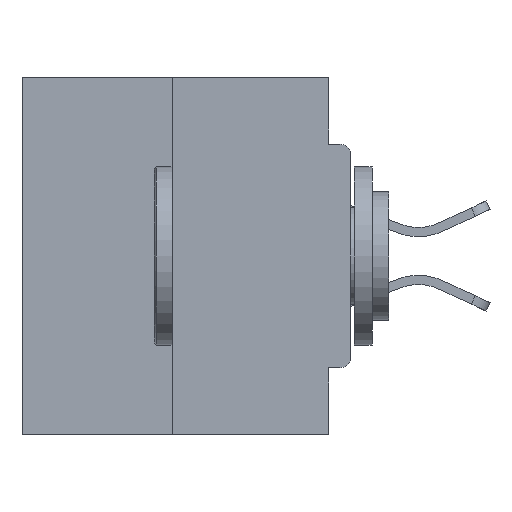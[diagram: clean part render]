
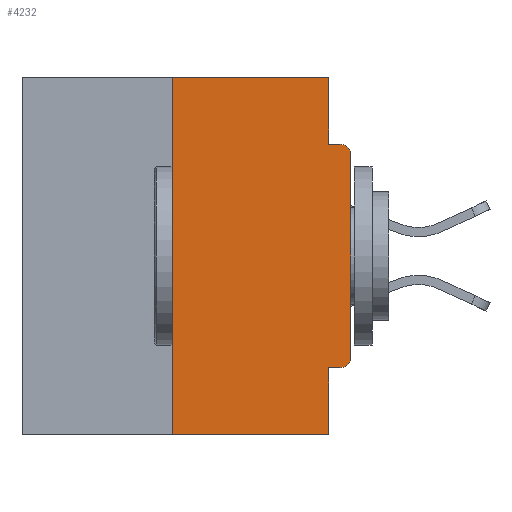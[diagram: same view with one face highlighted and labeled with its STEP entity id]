
A CAD part, left-side view. The second image highlights one B-rep face of the part: STEP entity #4232.
In plain terms, the highlighted planar face has unit normal (-1, 0, 0).
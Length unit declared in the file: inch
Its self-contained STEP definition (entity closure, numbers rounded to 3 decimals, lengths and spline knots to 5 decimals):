
#245 = FACE_OUTER_BOUND ( 'NONE', #23411, .T. ) ;
#441 = DIRECTION ( 'NONE',  ( 0., 0., -1. ) ) ;
#720 = CARTESIAN_POINT ( 'NONE',  ( 0., 0.25, 0. ) ) ;
#1564 = ORIENTED_EDGE ( 'NONE', *, *, #21520, .F. ) ;
#2626 = VERTEX_POINT ( 'NONE', #11842 ) ;
#3789 = CARTESIAN_POINT ( 'NONE',  ( 0., 0.25, 0. ) ) ;
#4232 = ADVANCED_FACE ( 'NONE', ( #245 ), #27365, .F. ) ;
#5403 = VECTOR ( 'NONE', #40375, 39.37008 ) ;
#5615 = VERTEX_POINT ( 'NONE', #6268 ) ;
#6268 = CARTESIAN_POINT ( 'NONE',  ( 0., 0.015, -0.0935 ) ) ;
#6535 = ORIENTED_EDGE ( 'NONE', *, *, #35798, .F. ) ;
#7224 = VECTOR ( 'NONE', #32529, 39.37008 ) ;
#7836 = CARTESIAN_POINT ( 'NONE',  ( 0., 0.031, 0. ) ) ;
#8249 = CARTESIAN_POINT ( 'NONE',  ( 0., 0.031, -0.5 ) ) ;
#8778 = LINE ( 'NONE', #10849, #42807 ) ;
#8936 = EDGE_CURVE ( 'NONE', #44453, #19351, #8778, .T. ) ;
#10328 = CARTESIAN_POINT ( 'NONE',  ( 0., 0.46, 0. ) ) ;
#10391 = CARTESIAN_POINT ( 'NONE',  ( 0., 0.46, -0.5 ) ) ;
#10849 = CARTESIAN_POINT ( 'NONE',  ( 0., 0.46, 0. ) ) ;
#11082 = ORIENTED_EDGE ( 'NONE', *, *, #35689, .F. ) ;
#11842 = CARTESIAN_POINT ( 'NONE',  ( 0., 0., -0.3915 ) ) ;
#11858 = DIRECTION ( 'NONE',  ( -1., 0., 0. ) ) ;
#12068 = ORIENTED_EDGE ( 'NONE', *, *, #8936, .F. ) ;
#12243 = VERTEX_POINT ( 'NONE', #24722 ) ;
#13790 = DIRECTION ( 'NONE',  ( 0., 0., -1. ) ) ;
#13841 = VERTEX_POINT ( 'NONE', #25505 ) ;
#13938 = ORIENTED_EDGE ( 'NONE', *, *, #21574, .F. ) ;
#14359 = VECTOR ( 'NONE', #35295, 39.37008 ) ;
#14517 = CARTESIAN_POINT ( 'NONE',  ( 0., 0., -0.1085 ) ) ;
#15699 = CARTESIAN_POINT ( 'NONE',  ( 0., 0.031, -0.0935 ) ) ;
#15742 = CARTESIAN_POINT ( 'NONE',  ( 0., 0.015, -0.1085 ) ) ;
#16186 = CARTESIAN_POINT ( 'NONE',  ( 0., 0., -0.4065 ) ) ;
#17304 = VERTEX_POINT ( 'NONE', #42454 ) ;
#17512 = CARTESIAN_POINT ( 'NONE',  ( 0., 0.015, -0.3915 ) ) ;
#17559 = VECTOR ( 'NONE', #32715, 39.37008 ) ;
#18458 = CIRCLE ( 'NONE', #26832, 0.015 ) ;
#18866 = LINE ( 'NONE', #24294, #37284 ) ;
#19076 = DIRECTION ( 'NONE',  ( 0., 0., 1. ) ) ;
#19351 = VERTEX_POINT ( 'NONE', #7836 ) ;
#20166 = LINE ( 'NONE', #8249, #7224 ) ;
#20228 = CARTESIAN_POINT ( 'NONE',  ( 0., 0.015, -0.4065 ) ) ;
#21520 = EDGE_CURVE ( 'NONE', #12243, #44453, #36477, .T. ) ;
#21574 = EDGE_CURVE ( 'NONE', #40465, #5615, #41922, .T. ) ;
#23272 = EDGE_CURVE ( 'NONE', #43516, #5615, #18458, .T. ) ;
#23411 = EDGE_LOOP ( 'NONE', ( #12068, #1564, #30266, #35054, #11082, #41819, #41011, #24442, #13938, #6535 ) ) ;
#24294 = CARTESIAN_POINT ( 'NONE',  ( 0., 0.031, 0. ) ) ;
#24442 = ORIENTED_EDGE ( 'NONE', *, *, #23272, .T. ) ;
#24722 = CARTESIAN_POINT ( 'NONE',  ( 0., 0.25, -0.5 ) ) ;
#25084 = LINE ( 'NONE', #36147, #26708 ) ;
#25365 = DIRECTION ( 'NONE',  ( 0., 0., -1. ) ) ;
#25505 = CARTESIAN_POINT ( 'NONE',  ( 0., 0.031, -0.5 ) ) ;
#26656 = EDGE_CURVE ( 'NONE', #2626, #43516, #25084, .T. ) ;
#26708 = VECTOR ( 'NONE', #19076, 39.37008 ) ;
#26832 = AXIS2_PLACEMENT_3D ( 'NONE', #15742, #11858, #43245 ) ;
#27365 = PLANE ( 'NONE',  #43199 ) ;
#27881 = VECTOR ( 'NONE', #30890, 39.37008 ) ;
#30266 = ORIENTED_EDGE ( 'NONE', *, *, #32606, .T. ) ;
#30684 = AXIS2_PLACEMENT_3D ( 'NONE', #17512, #38357, #441 ) ;
#30890 = DIRECTION ( 'NONE',  ( 0., -1., 0. ) ) ;
#31823 = CARTESIAN_POINT ( 'NONE',  ( 0., 0., -0.0935 ) ) ;
#32529 = DIRECTION ( 'NONE',  ( 0., 0., -1. ) ) ;
#32606 = EDGE_CURVE ( 'NONE', #12243, #13841, #43587, .T. ) ;
#32715 = DIRECTION ( 'NONE',  ( 0., -1., 0. ) ) ;
#33408 = EDGE_CURVE ( 'NONE', #17304, #13841, #20166, .T. ) ;
#33527 = CIRCLE ( 'NONE', #30684, 0.015 ) ;
#34154 = VERTEX_POINT ( 'NONE', #20228 ) ;
#34414 = DIRECTION ( 'NONE',  ( 1., 0., 0. ) ) ;
#35054 = ORIENTED_EDGE ( 'NONE', *, *, #33408, .F. ) ;
#35084 = EDGE_CURVE ( 'NONE', #34154, #2626, #33527, .T. ) ;
#35295 = DIRECTION ( 'NONE',  ( 0., 0., 1. ) ) ;
#35642 = LINE ( 'NONE', #16186, #5403 ) ;
#35689 = EDGE_CURVE ( 'NONE', #34154, #17304, #35642, .T. ) ;
#35798 = EDGE_CURVE ( 'NONE', #19351, #40465, #18866, .T. ) ;
#36147 = CARTESIAN_POINT ( 'NONE',  ( 0., 0., 0. ) ) ;
#36477 = LINE ( 'NONE', #720, #14359 ) ;
#37284 = VECTOR ( 'NONE', #25365, 39.37008 ) ;
#38276 = DIRECTION ( 'NONE',  ( 0., -1., 0. ) ) ;
#38357 = DIRECTION ( 'NONE',  ( -1., 0., 0. ) ) ;
#40375 = DIRECTION ( 'NONE',  ( 0., 1., 0. ) ) ;
#40465 = VERTEX_POINT ( 'NONE', #15699 ) ;
#41011 = ORIENTED_EDGE ( 'NONE', *, *, #26656, .T. ) ;
#41819 = ORIENTED_EDGE ( 'NONE', *, *, #35084, .T. ) ;
#41922 = LINE ( 'NONE', #31823, #17559 ) ;
#42454 = CARTESIAN_POINT ( 'NONE',  ( 0., 0.031, -0.4065 ) ) ;
#42807 = VECTOR ( 'NONE', #38276, 39.37008 ) ;
#43199 = AXIS2_PLACEMENT_3D ( 'NONE', #10328, #34414, #13790 ) ;
#43245 = DIRECTION ( 'NONE',  ( 0., 0., -1. ) ) ;
#43516 = VERTEX_POINT ( 'NONE', #14517 ) ;
#43587 = LINE ( 'NONE', #10391, #27881 ) ;
#44453 = VERTEX_POINT ( 'NONE', #3789 ) ;
